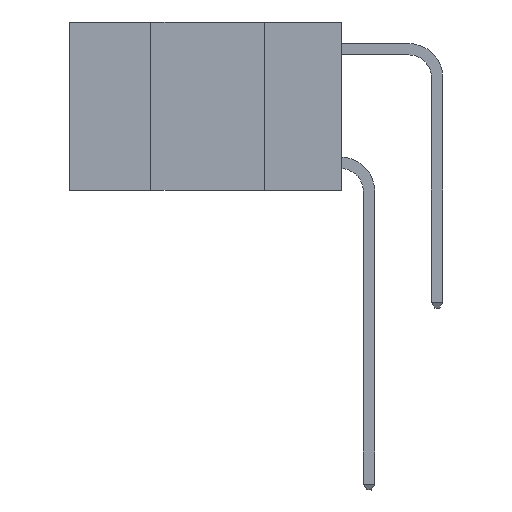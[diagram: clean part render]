
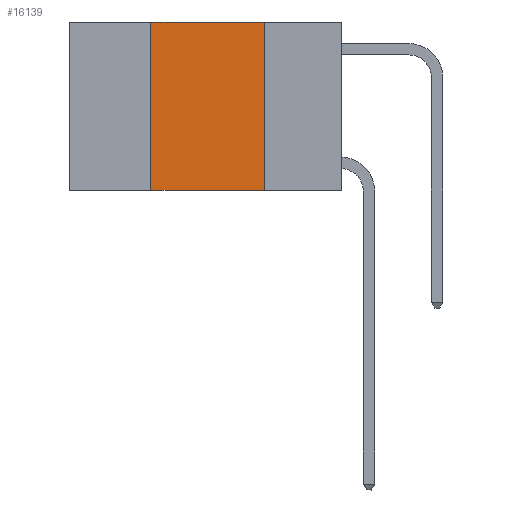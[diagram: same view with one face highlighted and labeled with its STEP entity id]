
A CAD part, left-side view. The second image highlights one B-rep face of the part: STEP entity #16139.
In plain terms, the highlighted planar face has unit normal (-1, 0, 0).
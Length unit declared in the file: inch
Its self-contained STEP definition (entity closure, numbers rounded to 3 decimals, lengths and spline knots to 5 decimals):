
#913 = DIRECTION ( 'NONE',  ( 0., 0., -1. ) ) ;
#1655 = CARTESIAN_POINT ( 'NONE',  ( 0., 0.42, 0. ) ) ;
#3259 = DIRECTION ( 'NONE',  ( 1., 0., 0. ) ) ;
#4197 = VECTOR ( 'NONE', #27289, 39.37008 ) ;
#4980 = EDGE_CURVE ( 'NONE', #7149, #16215, #4994, .T. ) ;
#4994 = LINE ( 'NONE', #29737, #24623 ) ;
#5015 = EDGE_CURVE ( 'NONE', #25109, #7149, #31435, .T. ) ;
#6056 = EDGE_CURVE ( 'NONE', #16215, #22310, #9325, .T. ) ;
#7149 = VERTEX_POINT ( 'NONE', #7430 ) ;
#7430 = CARTESIAN_POINT ( 'NONE',  ( 0., 0.42, 0. ) ) ;
#9114 = EDGE_CURVE ( 'NONE', #25109, #22310, #18344, .T. ) ;
#9325 = LINE ( 'NONE', #31585, #22145 ) ;
#11347 = ORIENTED_EDGE ( 'NONE', *, *, #6056, .F. ) ;
#13090 = ORIENTED_EDGE ( 'NONE', *, *, #9114, .T. ) ;
#15868 = ORIENTED_EDGE ( 'NONE', *, *, #5015, .F. ) ;
#16139 = ADVANCED_FACE ( 'NONE', ( #28655 ), #31348, .F. ) ;
#16215 = VERTEX_POINT ( 'NONE', #23947 ) ;
#16929 = CARTESIAN_POINT ( 'NONE',  ( 0., 0.6, -0.37 ) ) ;
#18344 = LINE ( 'NONE', #16929, #24377 ) ;
#18557 = CARTESIAN_POINT ( 'NONE',  ( 0., 0.6, 0. ) ) ;
#18818 = EDGE_LOOP ( 'NONE', ( #11347, #26270, #15868, #13090 ) ) ;
#20449 = DIRECTION ( 'NONE',  ( 0., -1., 0. ) ) ;
#21153 = DIRECTION ( 'NONE',  ( 0., 0., -1. ) ) ;
#22118 = DIRECTION ( 'NONE',  ( 0., -1., 0. ) ) ;
#22145 = VECTOR ( 'NONE', #913, 39.37008 ) ;
#22310 = VERTEX_POINT ( 'NONE', #23127 ) ;
#23127 = CARTESIAN_POINT ( 'NONE',  ( 0., 0.17, -0.37 ) ) ;
#23947 = CARTESIAN_POINT ( 'NONE',  ( 0., 0.17, 0. ) ) ;
#24377 = VECTOR ( 'NONE', #20449, 39.37008 ) ;
#24623 = VECTOR ( 'NONE', #22118, 39.37008 ) ;
#24950 = AXIS2_PLACEMENT_3D ( 'NONE', #18557, #3259, #21153 ) ;
#25109 = VERTEX_POINT ( 'NONE', #27677 ) ;
#26270 = ORIENTED_EDGE ( 'NONE', *, *, #4980, .F. ) ;
#27289 = DIRECTION ( 'NONE',  ( 0., 0., 1. ) ) ;
#27677 = CARTESIAN_POINT ( 'NONE',  ( 0., 0.42, -0.37 ) ) ;
#28655 = FACE_OUTER_BOUND ( 'NONE', #18818, .T. ) ;
#29737 = CARTESIAN_POINT ( 'NONE',  ( 0., 0.6, 0. ) ) ;
#31348 = PLANE ( 'NONE',  #24950 ) ;
#31435 = LINE ( 'NONE', #1655, #4197 ) ;
#31585 = CARTESIAN_POINT ( 'NONE',  ( 0., 0.17, 0. ) ) ;
